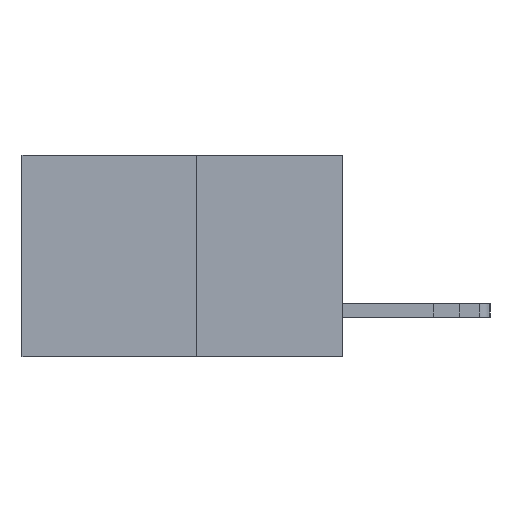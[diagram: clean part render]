
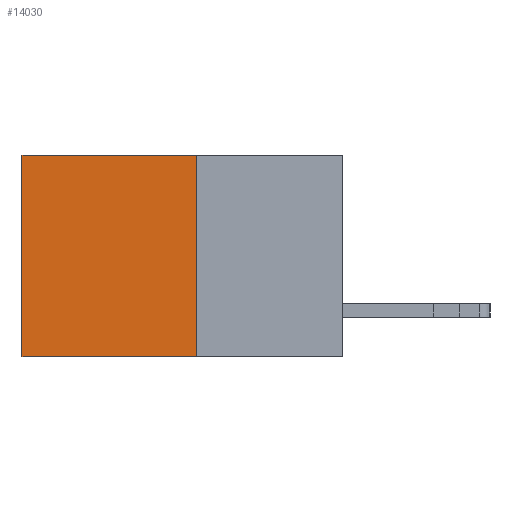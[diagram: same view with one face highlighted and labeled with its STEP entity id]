
A CAD part, left-side view. The second image highlights one B-rep face of the part: STEP entity #14030.
In plain terms, the highlighted planar face has unit normal (-1, 0, 0).
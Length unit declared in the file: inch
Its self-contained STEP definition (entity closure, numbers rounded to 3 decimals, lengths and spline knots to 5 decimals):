
#124 = DIRECTION ( 'NONE',  ( 0., 1., 0. ) ) ;
#653 = CARTESIAN_POINT ( 'NONE',  ( 0.277, 0.27, 0. ) ) ;
#724 = PLANE ( 'NONE',  #10259 ) ;
#937 = VERTEX_POINT ( 'NONE', #12040 ) ;
#1231 = LINE ( 'NONE', #653, #12811 ) ;
#1349 = VERTEX_POINT ( 'NONE', #7179 ) ;
#1392 = VERTEX_POINT ( 'NONE', #5964 ) ;
#1990 = DIRECTION ( 'NONE',  ( 1., 0., 0. ) ) ;
#2258 = VECTOR ( 'NONE', #13955, 39.37008 ) ;
#3722 = EDGE_CURVE ( 'NONE', #1392, #937, #11027, .T. ) ;
#5689 = EDGE_CURVE ( 'NONE', #1349, #1392, #1231, .T. ) ;
#5964 = CARTESIAN_POINT ( 'NONE',  ( 0.277, 0.59, 0. ) ) ;
#7179 = CARTESIAN_POINT ( 'NONE',  ( 0.277, 0.27, 0. ) ) ;
#7385 = VECTOR ( 'NONE', #7498, 39.37008 ) ;
#7410 = FACE_OUTER_BOUND ( 'NONE', #13245, .T. ) ;
#7498 = DIRECTION ( 'NONE',  ( 0., 1., 0. ) ) ;
#7644 = CARTESIAN_POINT ( 'NONE',  ( 0.277, 0.27, -0.37 ) ) ;
#8520 = EDGE_CURVE ( 'NONE', #1349, #14861, #9260, .T. ) ;
#9260 = LINE ( 'NONE', #12232, #11994 ) ;
#9703 = DIRECTION ( 'NONE',  ( 0., 0., -1. ) ) ;
#9863 = CARTESIAN_POINT ( 'NONE',  ( 0.277, 0.27, -0.37 ) ) ;
#10025 = DIRECTION ( 'NONE',  ( 0., 0., -1. ) ) ;
#10259 = AXIS2_PLACEMENT_3D ( 'NONE', #7644, #1990, #10025 ) ;
#10412 = EDGE_CURVE ( 'NONE', #14861, #937, #10502, .T. ) ;
#10502 = LINE ( 'NONE', #9863, #7385 ) ;
#11027 = LINE ( 'NONE', #12345, #2258 ) ;
#11994 = VECTOR ( 'NONE', #9703, 39.37008 ) ;
#12040 = CARTESIAN_POINT ( 'NONE',  ( 0.277, 0.59, -0.37 ) ) ;
#12232 = CARTESIAN_POINT ( 'NONE',  ( 0.277, 0.27, -0.37 ) ) ;
#12345 = CARTESIAN_POINT ( 'NONE',  ( 0.277, 0.59, -0.37 ) ) ;
#12811 = VECTOR ( 'NONE', #124, 39.37008 ) ;
#13245 = EDGE_LOOP ( 'NONE', ( #14339, #14544, #14561, #14850 ) ) ;
#13955 = DIRECTION ( 'NONE',  ( 0., 0., -1. ) ) ;
#14030 = ADVANCED_FACE ( 'NONE', ( #7410 ), #724, .F. ) ;
#14339 = ORIENTED_EDGE ( 'NONE', *, *, #3722, .T. ) ;
#14544 = ORIENTED_EDGE ( 'NONE', *, *, #10412, .F. ) ;
#14561 = ORIENTED_EDGE ( 'NONE', *, *, #8520, .F. ) ;
#14850 = ORIENTED_EDGE ( 'NONE', *, *, #5689, .T. ) ;
#14861 = VERTEX_POINT ( 'NONE', #14884 ) ;
#14884 = CARTESIAN_POINT ( 'NONE',  ( 0.277, 0.27, -0.37 ) ) ;
